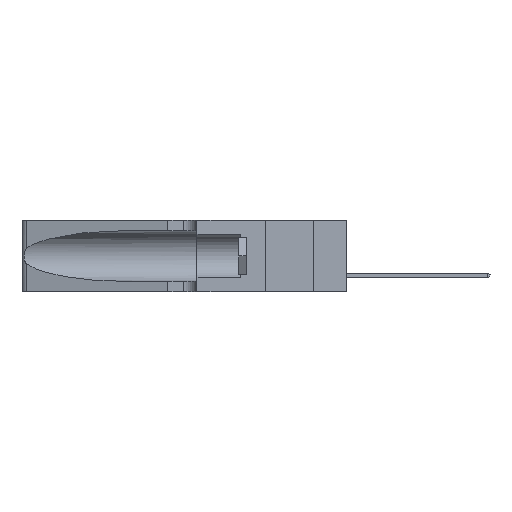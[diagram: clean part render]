
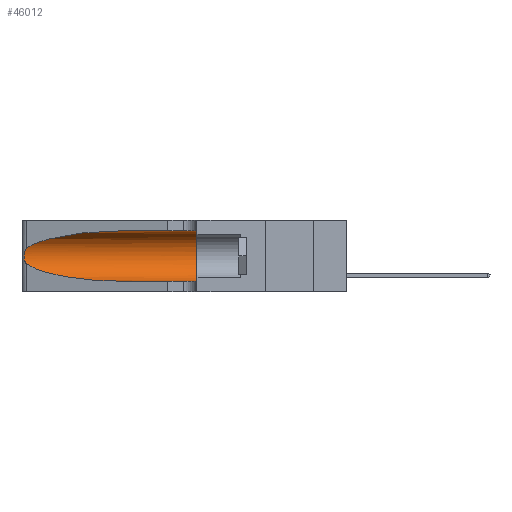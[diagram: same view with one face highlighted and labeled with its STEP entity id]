
A CAD part, left-side view. The second image highlights one B-rep face of the part: STEP entity #46012.
In plain terms, the highlighted cylindrical face has radius 3.308 mm (diameter 6.617 mm), a partial arc.
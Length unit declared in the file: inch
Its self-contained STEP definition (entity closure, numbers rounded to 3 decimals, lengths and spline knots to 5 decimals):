
#223 = DIRECTION ( 'NONE',  ( 0., -1., 0. ) ) ;
#2079 = DIRECTION ( 'NONE',  ( 0., -1., 0. ) ) ;
#4025 = VECTOR ( 'NONE', #20424, 39.37008 ) ;
#4323 = VERTEX_POINT ( 'NONE', #7264 ) ;
#4503 = CARTESIAN_POINT ( 'NONE',  ( 0.26075, 1.23896, 0.178 ) ) ;
#4697 = ORIENTED_EDGE ( 'NONE', *, *, #12728, .T. ) ;
#5923 = CARTESIAN_POINT ( 'NONE',  ( 0.25487, 1.22718, 0.14631 ) ) ;
#6031 = CARTESIAN_POINT ( 'NONE',  ( 0.2373, 1.15595, 0.28018 ) ) ;
#6762 = DIRECTION ( 'NONE',  ( 0., 0., 1. ) ) ;
#7264 = CARTESIAN_POINT ( 'NONE',  ( 0.25487, 1.22718, 0.22369 ) ) ;
#8061 = CARTESIAN_POINT ( 'NONE',  ( 0.26075, 1.23896, 0.19203 ) ) ;
#8875 = CARTESIAN_POINT ( 'NONE',  ( 0.1305, 0.35, 0.185 ) ) ;
#8991 = CARTESIAN_POINT ( 'NONE',  ( 0.1305, 0.72297, 0.31525 ) ) ;
#9894 = CARTESIAN_POINT ( 'NONE',  ( 0.2373, 1.15595, 0.08982 ) ) ;
#9992 = EDGE_CURVE ( 'NONE', #38984, #10385, #13729, .T. ) ;
#10156 = EDGE_CURVE ( 'NONE', #47351, #48651, #29126, .T. ) ;
#10385 = VERTEX_POINT ( 'NONE', #49239 ) ;
#12545 = EDGE_CURVE ( 'NONE', #48651, #41087, #42763, .T. ) ;
#12627 = CARTESIAN_POINT ( 'NONE',  ( 0.25789, 1.23486, 0.15765 ) ) ;
#12728 = EDGE_CURVE ( 'NONE', #4323, #38984, #16804, .T. ) ;
#13729 =( BOUNDED_CURVE ( )  B_SPLINE_CURVE ( 3, ( #5923, #9894, #25857, #36329 ),
 .UNSPECIFIED., .F., .F. ) 
 B_SPLINE_CURVE_WITH_KNOTS ( ( 4, 4 ),
 ( 3.44316, 4.71239 ),
 .UNSPECIFIED. ) 
 CURVE ( )  GEOMETRIC_REPRESENTATION_ITEM ( )  RATIONAL_B_SPLINE_CURVE ( ( 1., 0.87, 0.87, 1. ) ) 
 REPRESENTATION_ITEM ( '' )  );
#15436 = CARTESIAN_POINT ( 'NONE',  ( 0.25555, 1.22994, 0.2215 ) ) ;
#15748 = CYLINDRICAL_SURFACE ( 'NONE', #31086, 0.13025 ) ;
#16540 = CARTESIAN_POINT ( 'NONE',  ( 0.25487, 1.22718, 0.14631 ) ) ;
#16714 = CARTESIAN_POINT ( 'NONE',  ( 0.1305, 0.35, 0.05475 ) ) ;
#16804 = B_SPLINE_CURVE_WITH_KNOTS ( 'NONE', 3,
 ( #32595, #15436, #23288, #27640, #27169, #27315, #8061, #4503, #39650, #28303, #12627, #20736, #47526, #16540 ),
 .UNSPECIFIED., .F., .F.,
 ( 4, 2, 2, 2, 2, 2, 4 ),
 ( 0., 0.00027, 0.00053, 0.00107, 0.0016, 0.00187, 0.00214 ),
 .UNSPECIFIED. ) ;
#17332 = CARTESIAN_POINT ( 'NONE',  ( 0.25487, 1.22718, 0.22369 ) ) ;
#20424 = DIRECTION ( 'NONE',  ( 0., -1., 0. ) ) ;
#20736 = CARTESIAN_POINT ( 'NONE',  ( 0.25639, 1.23186, 0.15144 ) ) ;
#22112 = ORIENTED_EDGE ( 'NONE', *, *, #40027, .T. ) ;
#23288 = CARTESIAN_POINT ( 'NONE',  ( 0.25639, 1.23184, 0.21858 ) ) ;
#23512 = FACE_OUTER_BOUND ( 'NONE', #33206, .T. ) ;
#24143 = DIRECTION ( 'NONE',  ( 0., 0., -1. ) ) ;
#25857 = CARTESIAN_POINT ( 'NONE',  ( 0.18966, 0.96281, 0.05475 ) ) ;
#27169 = CARTESIAN_POINT ( 'NONE',  ( 0.25854, 1.2359, 0.20912 ) ) ;
#27315 = CARTESIAN_POINT ( 'NONE',  ( 0.26018, 1.23835, 0.19895 ) ) ;
#27640 = CARTESIAN_POINT ( 'NONE',  ( 0.25787, 1.23484, 0.2124 ) ) ;
#27677 = CARTESIAN_POINT ( 'NONE',  ( 0.1305, 1.61858, 0.05475 ) ) ;
#28303 = CARTESIAN_POINT ( 'NONE',  ( 0.25856, 1.23593, 0.16098 ) ) ;
#28899 = CARTESIAN_POINT ( 'NONE',  ( 0.1305, 0.72297, 0.31525 ) ) ;
#29010 = CARTESIAN_POINT ( 'NONE',  ( 0.25487, 1.22718, 0.14631 ) ) ;
#29126 = LINE ( 'NONE', #48660, #46547 ) ;
#29138 = ORIENTED_EDGE ( 'NONE', *, *, #36101, .T. ) ;
#31086 = AXIS2_PLACEMENT_3D ( 'NONE', #32094, #223, #24143 ) ;
#32094 = CARTESIAN_POINT ( 'NONE',  ( 0.1305, 1.61858, 0.185 ) ) ;
#32595 = CARTESIAN_POINT ( 'NONE',  ( 0.25487, 1.22718, 0.22369 ) ) ;
#33206 = EDGE_LOOP ( 'NONE', ( #22112, #4697, #39334, #29138, #44865, #47126 ) ) ;
#36101 = EDGE_CURVE ( 'NONE', #10385, #41087, #42114, .T. ) ;
#36329 = CARTESIAN_POINT ( 'NONE',  ( 0.1305, 0.72297, 0.05475 ) ) ;
#38984 = VERTEX_POINT ( 'NONE', #29010 ) ;
#39334 = ORIENTED_EDGE ( 'NONE', *, *, #9992, .T. ) ;
#39650 = CARTESIAN_POINT ( 'NONE',  ( 0.26017, 1.23833, 0.17102 ) ) ;
#40027 = EDGE_CURVE ( 'NONE', #47351, #4323, #49032, .T. ) ;
#40466 = CARTESIAN_POINT ( 'NONE',  ( 0.18966, 0.96281, 0.31525 ) ) ;
#41087 = VERTEX_POINT ( 'NONE', #16714 ) ;
#42114 = LINE ( 'NONE', #27677, #4025 ) ;
#42373 = AXIS2_PLACEMENT_3D ( 'NONE', #8875, #43692, #6762 ) ;
#42763 = CIRCLE ( 'NONE', #42373, 0.13025 ) ;
#43692 = DIRECTION ( 'NONE',  ( 0., 1., 0. ) ) ;
#44865 = ORIENTED_EDGE ( 'NONE', *, *, #12545, .F. ) ;
#46012 = ADVANCED_FACE ( 'NONE', ( #23512 ), #15748, .F. ) ;
#46547 = VECTOR ( 'NONE', #2079, 39.37008 ) ;
#47126 = ORIENTED_EDGE ( 'NONE', *, *, #10156, .F. ) ;
#47351 = VERTEX_POINT ( 'NONE', #28899 ) ;
#47526 = CARTESIAN_POINT ( 'NONE',  ( 0.25555, 1.22993, 0.14849 ) ) ;
#48651 = VERTEX_POINT ( 'NONE', #49047 ) ;
#48660 = CARTESIAN_POINT ( 'NONE',  ( 0.1305, 1.61858, 0.31525 ) ) ;
#49032 =( BOUNDED_CURVE ( )  B_SPLINE_CURVE ( 3, ( #8991, #40466, #6031, #17332 ),
 .UNSPECIFIED., .F., .T. ) 
 B_SPLINE_CURVE_WITH_KNOTS ( ( 4, 4 ),
 ( 1.5708, 2.84003 ),
 .UNSPECIFIED. ) 
 CURVE ( )  GEOMETRIC_REPRESENTATION_ITEM ( )  RATIONAL_B_SPLINE_CURVE ( ( 1., 0.87, 0.87, 1. ) ) 
 REPRESENTATION_ITEM ( '' )  );
#49047 = CARTESIAN_POINT ( 'NONE',  ( 0.1305, 0.35, 0.31525 ) ) ;
#49239 = CARTESIAN_POINT ( 'NONE',  ( 0.1305, 0.72297, 0.05475 ) ) ;
